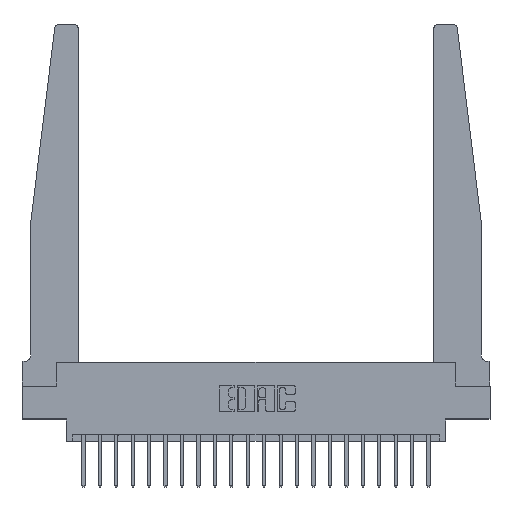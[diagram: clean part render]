
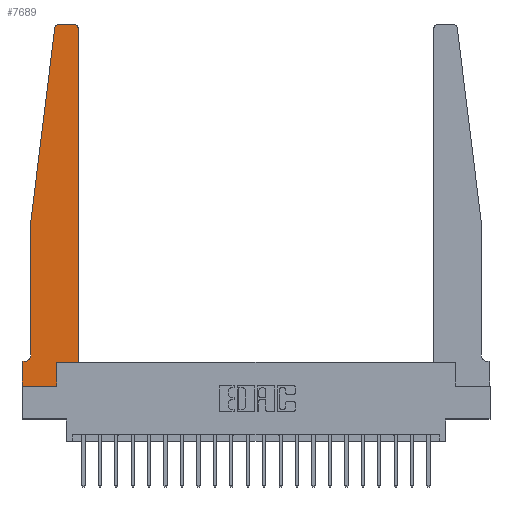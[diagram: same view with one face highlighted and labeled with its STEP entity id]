
A CAD part, top view. The second image highlights one B-rep face of the part: STEP entity #7689.
In plain terms, the highlighted planar face has unit normal (0, 0, 1).
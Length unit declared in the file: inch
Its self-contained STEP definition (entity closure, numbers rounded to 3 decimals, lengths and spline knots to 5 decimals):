
#62 = CARTESIAN_POINT ( 'NONE',  ( 0.015, 0.1875, 0.37 ) ) ;
#411 = AXIS2_PLACEMENT_3D ( 'NONE', #4065, #15983, #5790 ) ;
#675 = CARTESIAN_POINT ( 'NONE',  ( 0.065, 1.25, 0.37 ) ) ;
#682 = EDGE_CURVE ( 'NONE', #2127, #17737, #19060, .T. ) ;
#1199 = LINE ( 'NONE', #675, #14824 ) ;
#1543 = LINE ( 'NONE', #2869, #6611 ) ;
#1603 = AXIS2_PLACEMENT_3D ( 'NONE', #17029, #6866, #18713 ) ;
#1712 = ORIENTED_EDGE ( 'NONE', *, *, #18580, .T. ) ;
#1804 = CARTESIAN_POINT ( 'NONE',  ( 0., 0., 0.37 ) ) ;
#2111 = DIRECTION ( 'NONE',  ( 0., 0., 1. ) ) ;
#2127 = VERTEX_POINT ( 'NONE', #20637 ) ;
#2236 = EDGE_CURVE ( 'NONE', #17935, #6275, #14035, .T. ) ;
#2869 = CARTESIAN_POINT ( 'NONE',  ( 0.2605, 0.18, 0.37 ) ) ;
#3026 = VECTOR ( 'NONE', #20508, 39.37008 ) ;
#3053 = EDGE_CURVE ( 'NONE', #9468, #11411, #12683, .T. ) ;
#3202 = VECTOR ( 'NONE', #15435, 39.37008 ) ;
#3386 = VECTOR ( 'NONE', #11590, 39.37008 ) ;
#3635 = ORIENTED_EDGE ( 'NONE', *, *, #14989, .T. ) ;
#4065 = CARTESIAN_POINT ( 'NONE',  ( 0.395, 2.72, 0.37 ) ) ;
#4726 = ORIENTED_EDGE ( 'NONE', *, *, #10369, .T. ) ;
#5139 = DIRECTION ( 'NONE',  ( 1., 0., 0. ) ) ;
#5402 = CARTESIAN_POINT ( 'NONE',  ( 0., 0.1875, 0.37 ) ) ;
#5493 = ORIENTED_EDGE ( 'NONE', *, *, #3053, .T. ) ;
#5519 = ORIENTED_EDGE ( 'NONE', *, *, #13730, .T. ) ;
#5559 = VECTOR ( 'NONE', #9422, 39.37008 ) ;
#5790 = DIRECTION ( 'NONE',  ( 1., 0., 0. ) ) ;
#5863 = VERTEX_POINT ( 'NONE', #6264 ) ;
#5893 = CARTESIAN_POINT ( 'NONE',  ( 0.015, 0.2375, 0.37 ) ) ;
#6264 = CARTESIAN_POINT ( 'NONE',  ( 0.065, 1.25, 0.37 ) ) ;
#6275 = VERTEX_POINT ( 'NONE', #62 ) ;
#6386 = CARTESIAN_POINT ( 'NONE',  ( 0.065, 0.1875, 0.37 ) ) ;
#6568 = ORIENTED_EDGE ( 'NONE', *, *, #20813, .T. ) ;
#6611 = VECTOR ( 'NONE', #16472, 39.37008 ) ;
#6866 = DIRECTION ( 'NONE',  ( 0., 0., 1. ) ) ;
#7479 = DIRECTION ( 'NONE',  ( -0.122, -0.992, 0. ) ) ;
#7582 = VECTOR ( 'NONE', #16627, 39.37008 ) ;
#7608 = DIRECTION ( 'NONE',  ( -1., 0., 0. ) ) ;
#7619 = CARTESIAN_POINT ( 'NONE',  ( 0.24675, 2.72367, 0.37 ) ) ;
#7689 = ADVANCED_FACE ( 'NONE', ( #15279 ), #10649, .T. ) ;
#7951 = ORIENTED_EDGE ( 'NONE', *, *, #2236, .T. ) ;
#8348 = ORIENTED_EDGE ( 'NONE', *, *, #17332, .T. ) ;
#8354 = VERTEX_POINT ( 'NONE', #21061 ) ;
#8487 = CARTESIAN_POINT ( 'NONE',  ( 0., 0.1875, 0.37 ) ) ;
#8554 = CARTESIAN_POINT ( 'NONE',  ( 0., 0., 0.37 ) ) ;
#8650 = CARTESIAN_POINT ( 'NONE',  ( 0.065, 0.2375, 0.37 ) ) ;
#8664 = LINE ( 'NONE', #17006, #17138 ) ;
#9422 = DIRECTION ( 'NONE',  ( -1., 0., 0. ) ) ;
#9468 = VERTEX_POINT ( 'NONE', #21477 ) ;
#9691 = CARTESIAN_POINT ( 'NONE',  ( 0.2605, 0.18, 0.37 ) ) ;
#10320 = ORIENTED_EDGE ( 'NONE', *, *, #682, .T. ) ;
#10369 = EDGE_CURVE ( 'NONE', #18327, #20241, #12335, .T. ) ;
#10627 = AXIS2_PLACEMENT_3D ( 'NONE', #5402, #2111, #14057 ) ;
#10649 = PLANE ( 'NONE',  #10627 ) ;
#11327 = ORIENTED_EDGE ( 'NONE', *, *, #21267, .T. ) ;
#11411 = VERTEX_POINT ( 'NONE', #19565 ) ;
#11590 = DIRECTION ( 'NONE',  ( -1., 0., 0. ) ) ;
#11824 = EDGE_CURVE ( 'NONE', #5863, #17935, #12775, .T. ) ;
#11971 = LINE ( 'NONE', #6386, #3386 ) ;
#12159 = LINE ( 'NONE', #18796, #3026 ) ;
#12270 = VECTOR ( 'NONE', #15682, 39.37008 ) ;
#12335 = LINE ( 'NONE', #1804, #3202 ) ;
#12683 = LINE ( 'NONE', #14959, #7582 ) ;
#12775 = LINE ( 'NONE', #13994, #12270 ) ;
#13182 = CIRCLE ( 'NONE', #1603, 0.03 ) ;
#13281 = ORIENTED_EDGE ( 'NONE', *, *, #16312, .T. ) ;
#13517 = EDGE_LOOP ( 'NONE', ( #10320, #11327, #8348, #17311, #7951, #13281, #4726, #6568, #3635, #5519, #5493, #1712 ) ) ;
#13597 = CARTESIAN_POINT ( 'NONE',  ( 0.27653, 2.75, 0.37 ) ) ;
#13730 = EDGE_CURVE ( 'NONE', #14052, #9468, #8664, .T. ) ;
#13994 = CARTESIAN_POINT ( 'NONE',  ( 0.065, 1.25, 0.37 ) ) ;
#14035 = CIRCLE ( 'NONE', #18080, 0.05 ) ;
#14052 = VERTEX_POINT ( 'NONE', #9691 ) ;
#14057 = DIRECTION ( 'NONE',  ( 1., 0., 0. ) ) ;
#14824 = VECTOR ( 'NONE', #7479, 39.37008 ) ;
#14959 = CARTESIAN_POINT ( 'NONE',  ( 0.425, 0.18, 0.37 ) ) ;
#14989 = EDGE_CURVE ( 'NONE', #8354, #14052, #1543, .T. ) ;
#15279 = FACE_OUTER_BOUND ( 'NONE', #13517, .T. ) ;
#15435 = DIRECTION ( 'NONE',  ( 0., -1., 0. ) ) ;
#15539 = VERTEX_POINT ( 'NONE', #7619 ) ;
#15682 = DIRECTION ( 'NONE',  ( 0., -1., 0. ) ) ;
#15983 = DIRECTION ( 'NONE',  ( 0., 0., 1. ) ) ;
#16312 = EDGE_CURVE ( 'NONE', #6275, #18327, #11971, .T. ) ;
#16472 = DIRECTION ( 'NONE',  ( 0., 1., 0. ) ) ;
#16627 = DIRECTION ( 'NONE',  ( 0., 1., 0. ) ) ;
#17006 = CARTESIAN_POINT ( 'NONE',  ( 0.425, 0.18, 0.37 ) ) ;
#17029 = CARTESIAN_POINT ( 'NONE',  ( 0.27653, 2.72, 0.37 ) ) ;
#17138 = VECTOR ( 'NONE', #5139, 39.37008 ) ;
#17311 = ORIENTED_EDGE ( 'NONE', *, *, #11824, .T. ) ;
#17332 = EDGE_CURVE ( 'NONE', #15539, #5863, #1199, .T. ) ;
#17737 = VERTEX_POINT ( 'NONE', #13597 ) ;
#17748 = DIRECTION ( 'NONE',  ( 0., 0., -1. ) ) ;
#17935 = VERTEX_POINT ( 'NONE', #8650 ) ;
#18080 = AXIS2_PLACEMENT_3D ( 'NONE', #5893, #17748, #7608 ) ;
#18327 = VERTEX_POINT ( 'NONE', #8487 ) ;
#18424 = CIRCLE ( 'NONE', #411, 0.03 ) ;
#18580 = EDGE_CURVE ( 'NONE', #11411, #2127, #18424, .T. ) ;
#18713 = DIRECTION ( 'NONE',  ( 1., 0., 0. ) ) ;
#18796 = CARTESIAN_POINT ( 'NONE',  ( 0., 0., 0.37 ) ) ;
#19060 = LINE ( 'NONE', #19513, #5559 ) ;
#19513 = CARTESIAN_POINT ( 'NONE',  ( 0.25, 2.75, 0.37 ) ) ;
#19565 = CARTESIAN_POINT ( 'NONE',  ( 0.425, 2.72, 0.37 ) ) ;
#20241 = VERTEX_POINT ( 'NONE', #8554 ) ;
#20508 = DIRECTION ( 'NONE',  ( 1., 0., 0. ) ) ;
#20637 = CARTESIAN_POINT ( 'NONE',  ( 0.395, 2.75, 0.37 ) ) ;
#20813 = EDGE_CURVE ( 'NONE', #20241, #8354, #12159, .T. ) ;
#21061 = CARTESIAN_POINT ( 'NONE',  ( 0.2605, 0., 0.37 ) ) ;
#21267 = EDGE_CURVE ( 'NONE', #17737, #15539, #13182, .T. ) ;
#21477 = CARTESIAN_POINT ( 'NONE',  ( 0.425, 0.18, 0.37 ) ) ;
